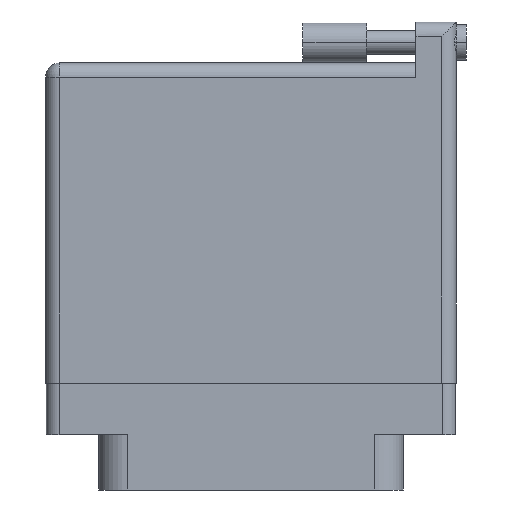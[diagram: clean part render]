
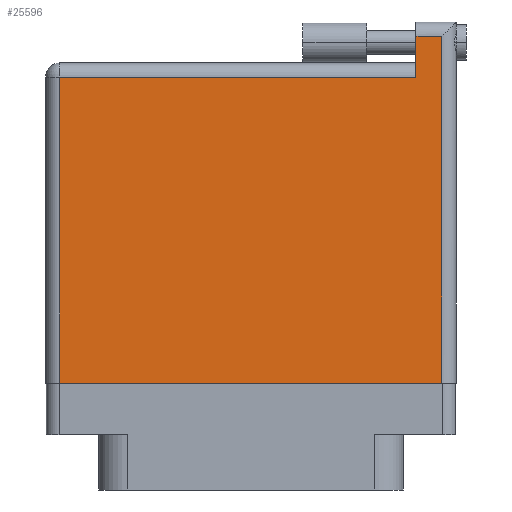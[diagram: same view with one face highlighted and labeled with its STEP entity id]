
A CAD part, front view. The second image highlights one B-rep face of the part: STEP entity #25596.
In plain terms, the highlighted face is planar.
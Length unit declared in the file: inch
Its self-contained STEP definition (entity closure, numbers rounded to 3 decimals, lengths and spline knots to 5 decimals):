
#532 = EDGE_CURVE ( 'NONE', #36864, #18563, #28159, .T. ) ;
#2999 = CARTESIAN_POINT ( 'NONE',  ( 0.934, 1.596, 0.4495 ) ) ;
#3026 = VECTOR ( 'NONE', #29314, 39.37008 ) ;
#3033 = LINE ( 'NONE', #12431, #19925 ) ;
#3146 = DIRECTION ( 'NONE',  ( 0., -1., 0. ) ) ;
#3875 = EDGE_LOOP ( 'NONE', ( #12182, #24390, #22701, #22836, #21510, #27544 ) ) ;
#3882 = DIRECTION ( 'NONE',  ( -1., 0., 0. ) ) ;
#4246 = DIRECTION ( 'NONE',  ( -1., 0., 0. ) ) ;
#4317 = DIRECTION ( 'NONE',  ( 1., 0., 0. ) ) ;
#4422 = CARTESIAN_POINT ( 'NONE',  ( 0.807, 1.596, 0.4495 ) ) ;
#4564 = AXIS2_PLACEMENT_3D ( 'NONE', #13009, #34939, #4246 ) ;
#4839 = VECTOR ( 'NONE', #4317, 39.37008 ) ;
#8541 = CARTESIAN_POINT ( 'NONE',  ( -0.934, 1.396, 0.4495 ) ) ;
#10497 = CARTESIAN_POINT ( 'NONE',  ( -1.004, -0.1, 0.4495 ) ) ;
#10793 = LINE ( 'NONE', #22455, #28578 ) ;
#11174 = VECTOR ( 'NONE', #3146, 39.37008 ) ;
#11763 = FACE_OUTER_BOUND ( 'NONE', #3875, .T. ) ;
#11955 = CARTESIAN_POINT ( 'NONE',  ( -0.934, -0.1, 0.4495 ) ) ;
#12007 = CARTESIAN_POINT ( 'NONE',  ( -0.934, -0.1, 0.4495 ) ) ;
#12182 = ORIENTED_EDGE ( 'NONE', *, *, #18819, .T. ) ;
#12431 = CARTESIAN_POINT ( 'NONE',  ( 0.934, 1.666, 0.4495 ) ) ;
#12954 = DIRECTION ( 'NONE',  ( 0., 1., 0. ) ) ;
#13009 = CARTESIAN_POINT ( 'NONE',  ( -1.004, 1.466, 0.4495 ) ) ;
#13199 = VECTOR ( 'NONE', #16089, 39.37008 ) ;
#13395 = PLANE ( 'NONE',  #4564 ) ;
#16089 = DIRECTION ( 'NONE',  ( 0., -1., 0. ) ) ;
#17151 = VERTEX_POINT ( 'NONE', #2999 ) ;
#18563 = VERTEX_POINT ( 'NONE', #12007 ) ;
#18819 = EDGE_CURVE ( 'NONE', #18563, #38860, #19728, .T. ) ;
#19728 = LINE ( 'NONE', #10497, #4839 ) ;
#19925 = VECTOR ( 'NONE', #12954, 39.37008 ) ;
#21285 = LINE ( 'NONE', #21568, #11174 ) ;
#21510 = ORIENTED_EDGE ( 'NONE', *, *, #39673, .T. ) ;
#21568 = CARTESIAN_POINT ( 'NONE',  ( 0.807, 1.666, 0.4495 ) ) ;
#22455 = CARTESIAN_POINT ( 'NONE',  ( -1.004, 1.596, 0.4495 ) ) ;
#22701 = ORIENTED_EDGE ( 'NONE', *, *, #31538, .T. ) ;
#22836 = ORIENTED_EDGE ( 'NONE', *, *, #24381, .T. ) ;
#24381 = EDGE_CURVE ( 'NONE', #27702, #36946, #21285, .T. ) ;
#24390 = ORIENTED_EDGE ( 'NONE', *, *, #26162, .T. ) ;
#24716 = CARTESIAN_POINT ( 'NONE',  ( 0.807, 1.396, 0.4495 ) ) ;
#25596 = ADVANCED_FACE ( 'NONE', ( #11763 ), #13395, .F. ) ;
#26162 = EDGE_CURVE ( 'NONE', #38860, #17151, #3033, .T. ) ;
#26228 = CARTESIAN_POINT ( 'NONE',  ( -1.004, 1.396, 0.4495 ) ) ;
#27544 = ORIENTED_EDGE ( 'NONE', *, *, #532, .T. ) ;
#27702 = VERTEX_POINT ( 'NONE', #4422 ) ;
#28061 = LINE ( 'NONE', #26228, #3026 ) ;
#28159 = LINE ( 'NONE', #11955, #13199 ) ;
#28578 = VECTOR ( 'NONE', #3882, 39.37008 ) ;
#29314 = DIRECTION ( 'NONE',  ( -1., 0., 0. ) ) ;
#30713 = CARTESIAN_POINT ( 'NONE',  ( 0.934, -0.1, 0.4495 ) ) ;
#31538 = EDGE_CURVE ( 'NONE', #17151, #27702, #10793, .T. ) ;
#34939 = DIRECTION ( 'NONE',  ( 0., 0., -1. ) ) ;
#36864 = VERTEX_POINT ( 'NONE', #8541 ) ;
#36946 = VERTEX_POINT ( 'NONE', #24716 ) ;
#38860 = VERTEX_POINT ( 'NONE', #30713 ) ;
#39673 = EDGE_CURVE ( 'NONE', #36946, #36864, #28061, .T. ) ;
